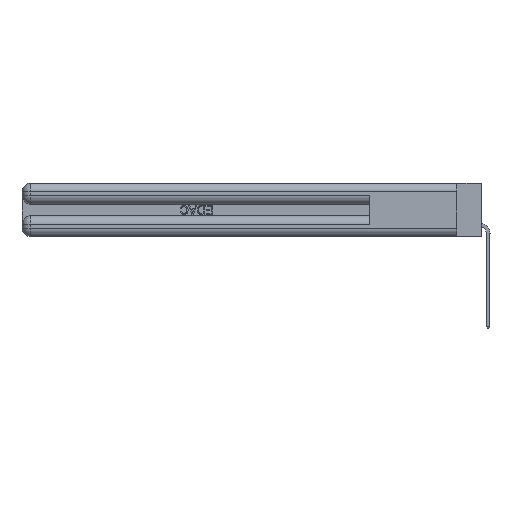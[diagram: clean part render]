
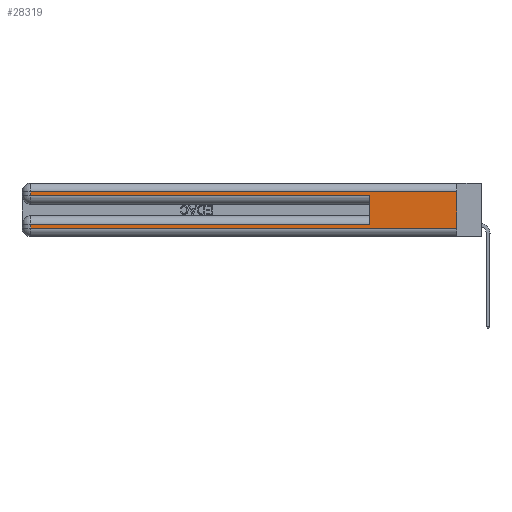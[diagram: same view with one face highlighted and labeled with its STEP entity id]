
A CAD part, left-side view. The second image highlights one B-rep face of the part: STEP entity #28319.
In plain terms, the highlighted planar face has unit normal (-1, 0, 0).
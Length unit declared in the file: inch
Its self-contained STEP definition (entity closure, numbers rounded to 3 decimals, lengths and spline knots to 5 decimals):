
#111 = EDGE_LOOP ( 'NONE', ( #23842, #12420, #25527, #6931, #16004, #21819, #43937, #2166 ) ) ;
#609 = CARTESIAN_POINT ( 'NONE',  ( 0., 2.94, 0.06 ) ) ;
#2166 = ORIENTED_EDGE ( 'NONE', *, *, #6000, .T. ) ;
#3591 = CARTESIAN_POINT ( 'NONE',  ( 0., 0., 0.31 ) ) ;
#4713 = DIRECTION ( 'NONE',  ( 0., 0., -1. ) ) ;
#5382 = CARTESIAN_POINT ( 'NONE',  ( 0., 0.6, 0.145 ) ) ;
#5510 = VERTEX_POINT ( 'NONE', #35646 ) ;
#5914 = CARTESIAN_POINT ( 'NONE',  ( 0., 2.94, 0.085 ) ) ;
#6000 = EDGE_CURVE ( 'NONE', #22214, #42012, #27062, .T. ) ;
#6931 = ORIENTED_EDGE ( 'NONE', *, *, #10590, .T. ) ;
#7767 = LINE ( 'NONE', #33001, #37179 ) ;
#8914 = EDGE_CURVE ( 'NONE', #17428, #22214, #47865, .T. ) ;
#10590 = EDGE_CURVE ( 'NONE', #47284, #24367, #42981, .T. ) ;
#10716 = EDGE_CURVE ( 'NONE', #5510, #17428, #43036, .T. ) ;
#11024 = CARTESIAN_POINT ( 'NONE',  ( 0., 0., 0.085 ) ) ;
#12420 = ORIENTED_EDGE ( 'NONE', *, *, #35688, .T. ) ;
#14216 = VECTOR ( 'NONE', #39117, 39.37008 ) ;
#15057 = CARTESIAN_POINT ( 'NONE',  ( 0., 0.6, 0.285 ) ) ;
#15451 = LINE ( 'NONE', #5382, #45507 ) ;
#16004 = ORIENTED_EDGE ( 'NONE', *, *, #16287, .F. ) ;
#16287 = EDGE_CURVE ( 'NONE', #5510, #24367, #15451, .T. ) ;
#17428 = VERTEX_POINT ( 'NONE', #5914 ) ;
#19849 = DIRECTION ( 'NONE',  ( 0., 1., 0. ) ) ;
#20650 = CARTESIAN_POINT ( 'NONE',  ( 0., 0., 0.06 ) ) ;
#21819 = ORIENTED_EDGE ( 'NONE', *, *, #10716, .T. ) ;
#22214 = VERTEX_POINT ( 'NONE', #609 ) ;
#23842 = ORIENTED_EDGE ( 'NONE', *, *, #27000, .F. ) ;
#24367 = VERTEX_POINT ( 'NONE', #15057 ) ;
#25004 = CARTESIAN_POINT ( 'NONE',  ( 0., 0., 0.37 ) ) ;
#25527 = ORIENTED_EDGE ( 'NONE', *, *, #43686, .T. ) ;
#25854 = VERTEX_POINT ( 'NONE', #31088 ) ;
#27000 = EDGE_CURVE ( 'NONE', #43350, #42012, #7767, .T. ) ;
#27062 = LINE ( 'NONE', #20650, #44212 ) ;
#27731 = DIRECTION ( 'NONE',  ( 0., 0., -1. ) ) ;
#28319 = ADVANCED_FACE ( 'NONE', ( #44094 ), #28761, .F. ) ;
#28498 = LINE ( 'NONE', #46132, #44974 ) ;
#28539 = DIRECTION ( 'NONE',  ( 0., 0., 1. ) ) ;
#28761 = PLANE ( 'NONE',  #37837 ) ;
#29023 = VECTOR ( 'NONE', #27731, 39.37008 ) ;
#29990 = VECTOR ( 'NONE', #19849, 39.37008 ) ;
#30688 = CARTESIAN_POINT ( 'NONE',  ( 0., 0., 0.31 ) ) ;
#31088 = CARTESIAN_POINT ( 'NONE',  ( 0., 2.94, 0.31 ) ) ;
#31641 = DIRECTION ( 'NONE',  ( 0., -1., 0. ) ) ;
#31727 = LINE ( 'NONE', #30688, #29990 ) ;
#32383 = DIRECTION ( 'NONE',  ( 0., 0., -1. ) ) ;
#33001 = CARTESIAN_POINT ( 'NONE',  ( 0., 0., 0.37 ) ) ;
#33053 = VECTOR ( 'NONE', #34488, 39.37008 ) ;
#33166 = DIRECTION ( 'NONE',  ( 0., 0., -1. ) ) ;
#33923 = CARTESIAN_POINT ( 'NONE',  ( 0., 2.94, 0.285 ) ) ;
#34488 = DIRECTION ( 'NONE',  ( 0., 1., 0. ) ) ;
#35646 = CARTESIAN_POINT ( 'NONE',  ( 0., 0.6, 0.085 ) ) ;
#35688 = EDGE_CURVE ( 'NONE', #43350, #25854, #31727, .T. ) ;
#36197 = DIRECTION ( 'NONE',  ( 1., 0., 0. ) ) ;
#37125 = CARTESIAN_POINT ( 'NONE',  ( 0., 0., 0.06 ) ) ;
#37179 = VECTOR ( 'NONE', #33166, 39.37008 ) ;
#37837 = AXIS2_PLACEMENT_3D ( 'NONE', #25004, #36197, #32383 ) ;
#39117 = DIRECTION ( 'NONE',  ( 0., -1., 0. ) ) ;
#42012 = VERTEX_POINT ( 'NONE', #37125 ) ;
#42712 = CARTESIAN_POINT ( 'NONE',  ( 0., 2.94, 0.37 ) ) ;
#42981 = LINE ( 'NONE', #46024, #14216 ) ;
#43036 = LINE ( 'NONE', #11024, #33053 ) ;
#43350 = VERTEX_POINT ( 'NONE', #3591 ) ;
#43686 = EDGE_CURVE ( 'NONE', #25854, #47284, #28498, .T. ) ;
#43937 = ORIENTED_EDGE ( 'NONE', *, *, #8914, .T. ) ;
#44094 = FACE_OUTER_BOUND ( 'NONE', #111, .T. ) ;
#44212 = VECTOR ( 'NONE', #31641, 39.37008 ) ;
#44974 = VECTOR ( 'NONE', #4713, 39.37008 ) ;
#45507 = VECTOR ( 'NONE', #28539, 39.37008 ) ;
#46024 = CARTESIAN_POINT ( 'NONE',  ( 0., 0., 0.285 ) ) ;
#46132 = CARTESIAN_POINT ( 'NONE',  ( 0., 2.94, 0.37 ) ) ;
#47284 = VERTEX_POINT ( 'NONE', #33923 ) ;
#47865 = LINE ( 'NONE', #42712, #29023 ) ;
